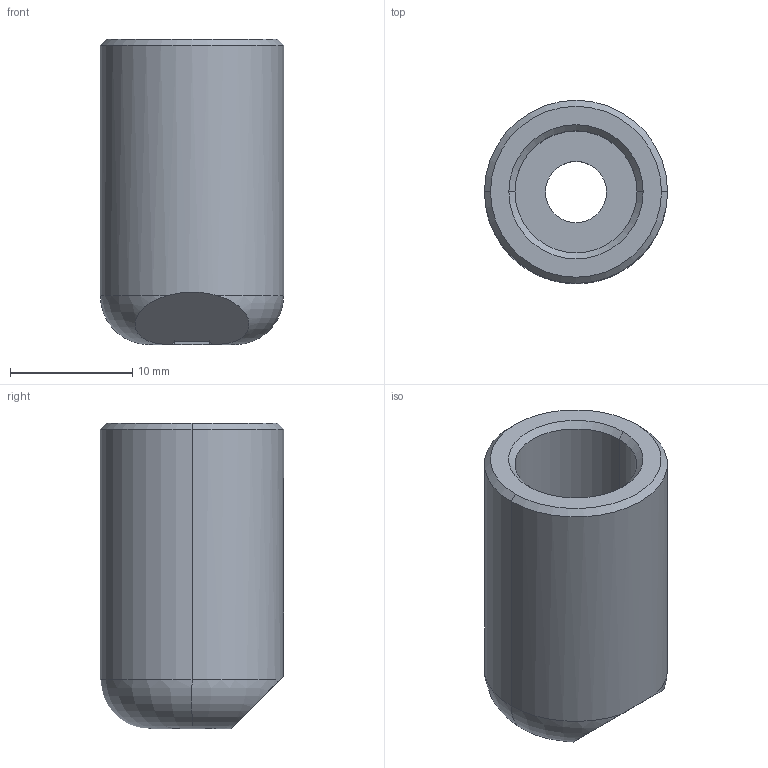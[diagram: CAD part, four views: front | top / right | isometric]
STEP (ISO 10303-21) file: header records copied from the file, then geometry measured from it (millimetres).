
FILE_DESCRIPTION (( 'STEP AP214' ), '1' );
FILE_NAME ('Charging Handle Short.step', '2019-12-18T03:07:27', ( '' ), ( '' ), 'SwSTEP 2.0', 'SolidWorks 2019', '' );
FILE_SCHEMA (( 'AUTOMOTIVE_DESIGN' ));
Length unit declared in the file: millimetre
Products named in the file (1): Charging Handle Short
Bounding box: 15 x 15 x 25 mm (x, y, z)
Volume: 2825.2 mm3; surface area: 2029.5 mm2
Topology: 1 solids, 1 shells, 25 faces, 60 edges, 38 vertices
Faces by surface type: plane 12, cylinder 6, cone 4, torus 3
Entity records: 826 total; most frequent: CARTESIAN_POINT 212, ORIENTED_EDGE 120, DIRECTION 119, EDGE_CURVE 60, AXIS2_PLACEMENT_3D 45, VERTEX_POINT 38, LINE 29, VECTOR 29
